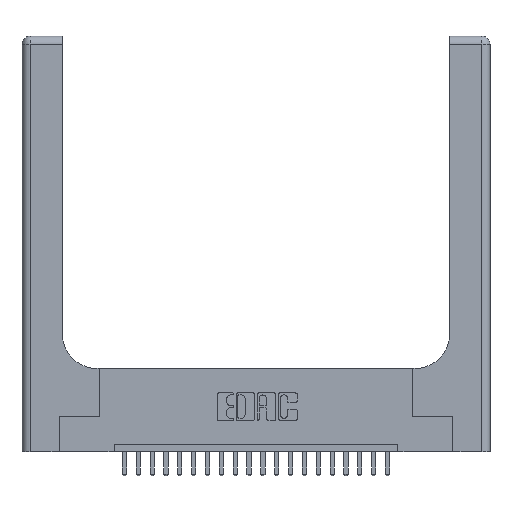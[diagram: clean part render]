
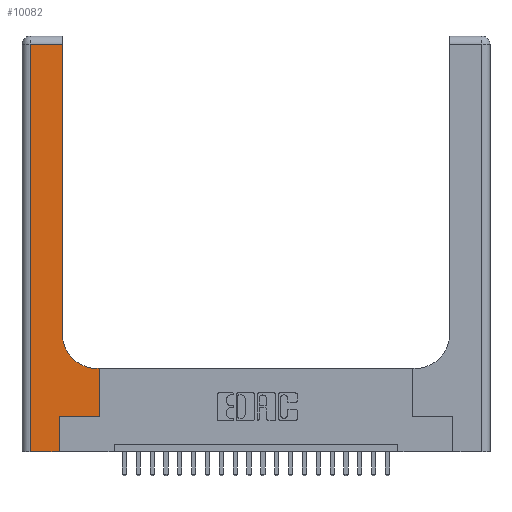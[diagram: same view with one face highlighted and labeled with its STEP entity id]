
A CAD part, top view. The second image highlights one B-rep face of the part: STEP entity #10082.
In plain terms, the highlighted planar face has unit normal (0, 0, 1).
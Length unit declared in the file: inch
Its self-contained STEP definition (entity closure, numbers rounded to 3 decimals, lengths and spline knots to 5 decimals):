
#469 = VERTEX_POINT ( 'NONE', #14123 ) ;
#599 = DIRECTION ( 'NONE',  ( 0., -1., 0. ) ) ;
#1221 = EDGE_CURVE ( 'NONE', #20855, #5217, #17465, .T. ) ;
#2885 = VECTOR ( 'NONE', #3567, 39.37008 ) ;
#3567 = DIRECTION ( 'NONE',  ( 1., 0., 0. ) ) ;
#3704 = CARTESIAN_POINT ( 'NONE',  ( 0.2915, 0.6, 0.37 ) ) ;
#3871 = DIRECTION ( 'NONE',  ( 1., 0., 0. ) ) ;
#3915 = ORIENTED_EDGE ( 'NONE', *, *, #15073, .T. ) ;
#4580 = LINE ( 'NONE', #16144, #17526 ) ;
#4589 = VERTEX_POINT ( 'NONE', #22452 ) ;
#5217 = VERTEX_POINT ( 'NONE', #21357 ) ;
#5418 = CARTESIAN_POINT ( 'NONE',  ( 0.5585, 0.6, 0.37 ) ) ;
#5600 = VERTEX_POINT ( 'NONE', #8173 ) ;
#5691 = ORIENTED_EDGE ( 'NONE', *, *, #6310, .T. ) ;
#6070 = VECTOR ( 'NONE', #18195, 39.37008 ) ;
#6310 = EDGE_CURVE ( 'NONE', #21193, #4589, #12829, .T. ) ;
#6438 = ORIENTED_EDGE ( 'NONE', *, *, #23205, .T. ) ;
#6672 = ORIENTED_EDGE ( 'NONE', *, *, #19732, .T. ) ;
#6895 = CARTESIAN_POINT ( 'NONE',  ( 0.269, 0., 0.37 ) ) ;
#6970 = CARTESIAN_POINT ( 'NONE',  ( 0.269, 0., 0.37 ) ) ;
#6985 = AXIS2_PLACEMENT_3D ( 'NONE', #9804, #20286, #7843 ) ;
#7635 = CARTESIAN_POINT ( 'NONE',  ( 0.06, 3., 0.37 ) ) ;
#7777 = CARTESIAN_POINT ( 'NONE',  ( 0., 3., 0.37 ) ) ;
#7843 = DIRECTION ( 'NONE',  ( 1., 0., 0. ) ) ;
#8173 = CARTESIAN_POINT ( 'NONE',  ( 0.5585, 0.25, 0.37 ) ) ;
#9804 = CARTESIAN_POINT ( 'NONE',  ( 0.5415, 0.85, 0.37 ) ) ;
#9905 = VERTEX_POINT ( 'NONE', #15909 ) ;
#10082 = ADVANCED_FACE ( 'NONE', ( #21698 ), #18548, .F. ) ;
#10166 = VECTOR ( 'NONE', #13978, 39.37008 ) ;
#10500 = DIRECTION ( 'NONE',  ( 0., 1., 0. ) ) ;
#11132 = VERTEX_POINT ( 'NONE', #5418 ) ;
#11304 = AXIS2_PLACEMENT_3D ( 'NONE', #7777, #22157, #14970 ) ;
#11414 = LINE ( 'NONE', #3704, #13356 ) ;
#11810 = EDGE_LOOP ( 'NONE', ( #21099, #19007, #6672, #19084, #5691, #14908, #19249, #6438, #3915 ) ) ;
#12755 = EDGE_CURVE ( 'NONE', #4589, #5600, #14718, .T. ) ;
#12769 = CARTESIAN_POINT ( 'NONE',  ( 0., 2.94, 0.37 ) ) ;
#12829 = LINE ( 'NONE', #6895, #19050 ) ;
#12969 = CARTESIAN_POINT ( 'NONE',  ( 0.2915, 0.85, 0.37 ) ) ;
#13348 = VERTEX_POINT ( 'NONE', #23101 ) ;
#13356 = VECTOR ( 'NONE', #20117, 39.37008 ) ;
#13873 = EDGE_CURVE ( 'NONE', #13348, #21193, #16022, .T. ) ;
#13978 = DIRECTION ( 'NONE',  ( 0., 1., 0. ) ) ;
#14123 = CARTESIAN_POINT ( 'NONE',  ( 0.5415, 0.6, 0.37 ) ) ;
#14718 = LINE ( 'NONE', #15670, #2885 ) ;
#14908 = ORIENTED_EDGE ( 'NONE', *, *, #12755, .T. ) ;
#14970 = DIRECTION ( 'NONE',  ( -1., 0., 0. ) ) ;
#15073 = EDGE_CURVE ( 'NONE', #469, #20855, #21080, .T. ) ;
#15670 = CARTESIAN_POINT ( 'NONE',  ( 0.269, 0.25, 0.37 ) ) ;
#15897 = DIRECTION ( 'NONE',  ( 0., 1., 0. ) ) ;
#15909 = CARTESIAN_POINT ( 'NONE',  ( 0.06, 2.94, 0.37 ) ) ;
#16022 = LINE ( 'NONE', #20033, #21984 ) ;
#16144 = CARTESIAN_POINT ( 'NONE',  ( 0.5585, 0.25, 0.37 ) ) ;
#17097 = EDGE_CURVE ( 'NONE', #5217, #9905, #17590, .T. ) ;
#17465 = LINE ( 'NONE', #19366, #10166 ) ;
#17526 = VECTOR ( 'NONE', #15897, 39.37008 ) ;
#17590 = LINE ( 'NONE', #12769, #6070 ) ;
#18195 = DIRECTION ( 'NONE',  ( -1., 0., 0. ) ) ;
#18197 = EDGE_CURVE ( 'NONE', #5600, #11132, #4580, .T. ) ;
#18548 = PLANE ( 'NONE',  #11304 ) ;
#18633 = LINE ( 'NONE', #7635, #22836 ) ;
#19007 = ORIENTED_EDGE ( 'NONE', *, *, #17097, .T. ) ;
#19050 = VECTOR ( 'NONE', #10500, 39.37008 ) ;
#19084 = ORIENTED_EDGE ( 'NONE', *, *, #13873, .T. ) ;
#19249 = ORIENTED_EDGE ( 'NONE', *, *, #18197, .T. ) ;
#19366 = CARTESIAN_POINT ( 'NONE',  ( 0.2915, 3., 0.37 ) ) ;
#19732 = EDGE_CURVE ( 'NONE', #9905, #13348, #18633, .T. ) ;
#20033 = CARTESIAN_POINT ( 'NONE',  ( 0., 0., 0.37 ) ) ;
#20117 = DIRECTION ( 'NONE',  ( -1., 0., 0. ) ) ;
#20286 = DIRECTION ( 'NONE',  ( 0., 0., -1. ) ) ;
#20855 = VERTEX_POINT ( 'NONE', #12969 ) ;
#21080 = CIRCLE ( 'NONE', #6985, 0.25 ) ;
#21099 = ORIENTED_EDGE ( 'NONE', *, *, #1221, .T. ) ;
#21193 = VERTEX_POINT ( 'NONE', #6970 ) ;
#21357 = CARTESIAN_POINT ( 'NONE',  ( 0.2915, 2.94, 0.37 ) ) ;
#21698 = FACE_OUTER_BOUND ( 'NONE', #11810, .T. ) ;
#21984 = VECTOR ( 'NONE', #3871, 39.37008 ) ;
#22157 = DIRECTION ( 'NONE',  ( 0., 0., -1. ) ) ;
#22452 = CARTESIAN_POINT ( 'NONE',  ( 0.269, 0.25, 0.37 ) ) ;
#22836 = VECTOR ( 'NONE', #599, 39.37008 ) ;
#23101 = CARTESIAN_POINT ( 'NONE',  ( 0.06, 0., 0.37 ) ) ;
#23205 = EDGE_CURVE ( 'NONE', #11132, #469, #11414, .T. ) ;
